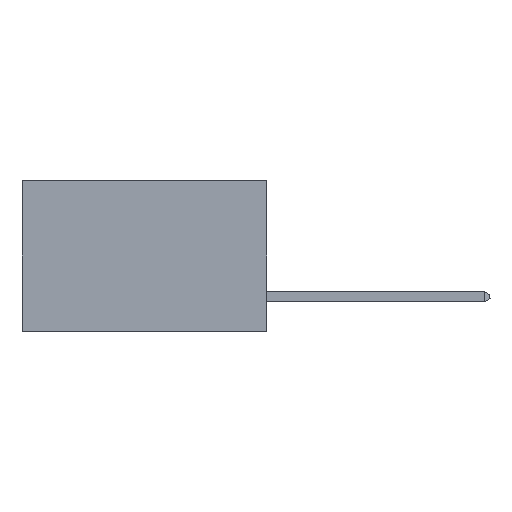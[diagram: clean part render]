
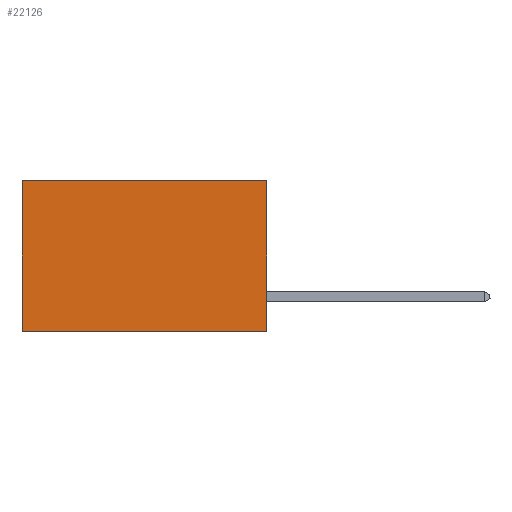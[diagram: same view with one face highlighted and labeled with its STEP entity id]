
A CAD part, left-side view. The second image highlights one B-rep face of the part: STEP entity #22126.
In plain terms, the highlighted planar face has unit normal (-1, 0, 0).
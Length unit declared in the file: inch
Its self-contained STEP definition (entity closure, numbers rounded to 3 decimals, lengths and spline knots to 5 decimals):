
#1036 = CARTESIAN_POINT ( 'NONE',  ( 0.2875, 0.6, 0. ) ) ;
#4122 = EDGE_CURVE ( 'NONE', #13800, #33603, #21440, .T. ) ;
#4503 = ORIENTED_EDGE ( 'NONE', *, *, #19146, .T. ) ;
#5026 = PLANE ( 'NONE',  #21952 ) ;
#5347 = CARTESIAN_POINT ( 'NONE',  ( 0.2875, 0., 0. ) ) ;
#5732 = CARTESIAN_POINT ( 'NONE',  ( 0.2875, 0.6, -0.37 ) ) ;
#7710 = CARTESIAN_POINT ( 'NONE',  ( 0.2875, 0., -0.37 ) ) ;
#7826 = EDGE_CURVE ( 'NONE', #16530, #19980, #16068, .T. ) ;
#9819 = DIRECTION ( 'NONE',  ( 0., 0., -1. ) ) ;
#9919 = DIRECTION ( 'NONE',  ( 0., 0., -1. ) ) ;
#10305 = ORIENTED_EDGE ( 'NONE', *, *, #4122, .F. ) ;
#11079 = LINE ( 'NONE', #7710, #21904 ) ;
#12357 = ORIENTED_EDGE ( 'NONE', *, *, #7826, .T. ) ;
#12707 = DIRECTION ( 'NONE',  ( 0., 1., 0. ) ) ;
#12966 = VECTOR ( 'NONE', #12707, 39.37008 ) ;
#13072 = VECTOR ( 'NONE', #9919, 39.37008 ) ;
#13800 = VERTEX_POINT ( 'NONE', #16315 ) ;
#14490 = DIRECTION ( 'NONE',  ( 1., 0., 0. ) ) ;
#14743 = FACE_OUTER_BOUND ( 'NONE', #29336, .T. ) ;
#14904 = DIRECTION ( 'NONE',  ( 0., 0., -1. ) ) ;
#14983 = ORIENTED_EDGE ( 'NONE', *, *, #16318, .F. ) ;
#16068 = LINE ( 'NONE', #1036, #13072 ) ;
#16315 = CARTESIAN_POINT ( 'NONE',  ( 0.2875, 0., 0. ) ) ;
#16318 = EDGE_CURVE ( 'NONE', #33603, #19980, #11079, .T. ) ;
#16530 = VERTEX_POINT ( 'NONE', #31846 ) ;
#19146 = EDGE_CURVE ( 'NONE', #13800, #16530, #21359, .T. ) ;
#19980 = VERTEX_POINT ( 'NONE', #5732 ) ;
#21359 = LINE ( 'NONE', #34266, #12966 ) ;
#21440 = LINE ( 'NONE', #5347, #37149 ) ;
#21904 = VECTOR ( 'NONE', #23235, 39.37008 ) ;
#21952 = AXIS2_PLACEMENT_3D ( 'NONE', #33244, #14490, #14904 ) ;
#22126 = ADVANCED_FACE ( 'NONE', ( #14743 ), #5026, .F. ) ;
#23235 = DIRECTION ( 'NONE',  ( 0., 1., 0. ) ) ;
#27375 = CARTESIAN_POINT ( 'NONE',  ( 0.2875, 0., -0.37 ) ) ;
#29336 = EDGE_LOOP ( 'NONE', ( #12357, #14983, #10305, #4503 ) ) ;
#31846 = CARTESIAN_POINT ( 'NONE',  ( 0.2875, 0.6, 0. ) ) ;
#33244 = CARTESIAN_POINT ( 'NONE',  ( 0.2875, 0., 0. ) ) ;
#33603 = VERTEX_POINT ( 'NONE', #27375 ) ;
#34266 = CARTESIAN_POINT ( 'NONE',  ( 0.2875, 0., 0. ) ) ;
#37149 = VECTOR ( 'NONE', #9819, 39.37008 ) ;
